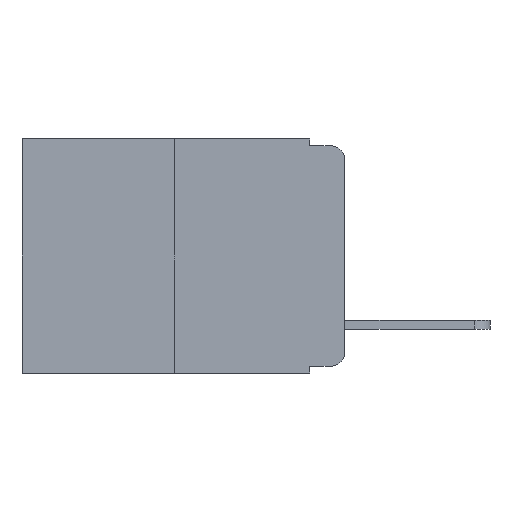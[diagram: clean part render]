
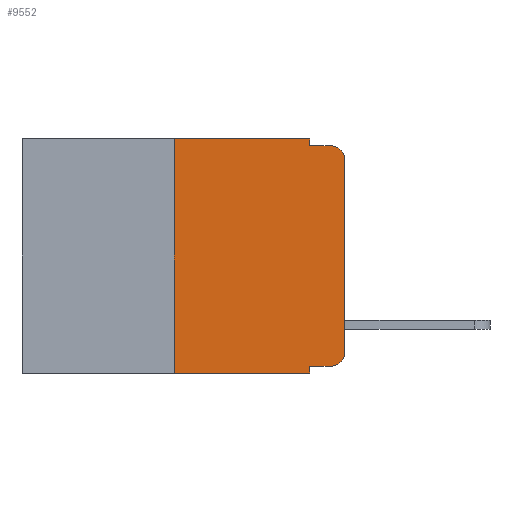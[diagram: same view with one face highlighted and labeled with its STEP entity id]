
A CAD part, left-side view. The second image highlights one B-rep face of the part: STEP entity #9552.
In plain terms, the highlighted planar face has unit normal (-1, 0, 0).
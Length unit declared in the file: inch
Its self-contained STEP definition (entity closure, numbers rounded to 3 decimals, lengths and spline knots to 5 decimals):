
#136 = LINE ( 'NONE', #9930, #23091 ) ;
#436 = CARTESIAN_POINT ( 'NONE',  ( 0., 0.02, -0.333 ) ) ;
#483 = CIRCLE ( 'NONE', #1491, 0.02 ) ;
#1447 = CARTESIAN_POINT ( 'NONE',  ( 0., 0.051, 0. ) ) ;
#1491 = AXIS2_PLACEMENT_3D ( 'NONE', #12486, #14298, #22160 ) ;
#2472 = DIRECTION ( 'NONE',  ( 0., 0., -1. ) ) ;
#2487 = LINE ( 'NONE', #19774, #5887 ) ;
#2876 = VERTEX_POINT ( 'NONE', #5480 ) ;
#3616 = FACE_OUTER_BOUND ( 'NONE', #20516, .T. ) ;
#3927 = VECTOR ( 'NONE', #20649, 39.37008 ) ;
#4208 = VECTOR ( 'NONE', #23397, 39.37008 ) ;
#4296 = EDGE_CURVE ( 'NONE', #2876, #12382, #16126, .T. ) ;
#4303 = DIRECTION ( 'NONE',  ( 0., -1., 0. ) ) ;
#4790 = ORIENTED_EDGE ( 'NONE', *, *, #22300, .F. ) ;
#5338 = CARTESIAN_POINT ( 'NONE',  ( 0., 0.051, -0.01 ) ) ;
#5480 = CARTESIAN_POINT ( 'NONE',  ( 0., 0.051, -0.333 ) ) ;
#5854 = ORIENTED_EDGE ( 'NONE', *, *, #10366, .T. ) ;
#5887 = VECTOR ( 'NONE', #6390, 39.37008 ) ;
#6390 = DIRECTION ( 'NONE',  ( 0., 0., 1. ) ) ;
#6560 = VERTEX_POINT ( 'NONE', #24103 ) ;
#7175 = EDGE_CURVE ( 'NONE', #20776, #17147, #11978, .T. ) ;
#7415 = LINE ( 'NONE', #9196, #9282 ) ;
#7894 = ORIENTED_EDGE ( 'NONE', *, *, #12988, .F. ) ;
#8194 = DIRECTION ( 'NONE',  ( 0., 0., -1. ) ) ;
#8550 = ORIENTED_EDGE ( 'NONE', *, *, #25464, .T. ) ;
#9196 = CARTESIAN_POINT ( 'NONE',  ( 0., 0., 0. ) ) ;
#9223 = CIRCLE ( 'NONE', #21379, 0.02 ) ;
#9281 = CARTESIAN_POINT ( 'NONE',  ( 0., 0.25, 0. ) ) ;
#9282 = VECTOR ( 'NONE', #9374, 39.37008 ) ;
#9374 = DIRECTION ( 'NONE',  ( 0., 0., 1. ) ) ;
#9552 = ADVANCED_FACE ( 'NONE', ( #3616 ), #20704, .F. ) ;
#9930 = CARTESIAN_POINT ( 'NONE',  ( 0., 0.473, -0.343 ) ) ;
#10149 = ORIENTED_EDGE ( 'NONE', *, *, #22702, .T. ) ;
#10366 = EDGE_CURVE ( 'NONE', #14837, #18911, #483, .T. ) ;
#10436 = ORIENTED_EDGE ( 'NONE', *, *, #13458, .T. ) ;
#10779 = CARTESIAN_POINT ( 'NONE',  ( 0., 0.473, 0. ) ) ;
#11978 = LINE ( 'NONE', #23557, #4208 ) ;
#12382 = VERTEX_POINT ( 'NONE', #436 ) ;
#12486 = CARTESIAN_POINT ( 'NONE',  ( 0., 0.02, -0.03 ) ) ;
#12988 = EDGE_CURVE ( 'NONE', #25314, #23221, #2487, .T. ) ;
#13236 = CARTESIAN_POINT ( 'NONE',  ( 0., 0.02, -0.01 ) ) ;
#13458 = EDGE_CURVE ( 'NONE', #6560, #14837, #7415, .T. ) ;
#14298 = DIRECTION ( 'NONE',  ( -1., 0., 0. ) ) ;
#14602 = EDGE_CURVE ( 'NONE', #17147, #18911, #16035, .T. ) ;
#14837 = VERTEX_POINT ( 'NONE', #23226 ) ;
#15304 = ORIENTED_EDGE ( 'NONE', *, *, #7175, .F. ) ;
#15762 = LINE ( 'NONE', #24044, #21383 ) ;
#15894 = CARTESIAN_POINT ( 'NONE',  ( 0., 0.051, -0.343 ) ) ;
#15936 = ORIENTED_EDGE ( 'NONE', *, *, #4296, .T. ) ;
#16035 = LINE ( 'NONE', #16439, #3927 ) ;
#16126 = LINE ( 'NONE', #24629, #20848 ) ;
#16286 = VERTEX_POINT ( 'NONE', #15894 ) ;
#16367 = ORIENTED_EDGE ( 'NONE', *, *, #21676, .F. ) ;
#16439 = CARTESIAN_POINT ( 'NONE',  ( 0., 0.051, -0.01 ) ) ;
#17147 = VERTEX_POINT ( 'NONE', #5338 ) ;
#18271 = VECTOR ( 'NONE', #4303, 39.37008 ) ;
#18911 = VERTEX_POINT ( 'NONE', #13236 ) ;
#19643 = CARTESIAN_POINT ( 'NONE',  ( 0., 0.02, -0.313 ) ) ;
#19774 = CARTESIAN_POINT ( 'NONE',  ( 0., 0.25, 0. ) ) ;
#20014 = DIRECTION ( 'NONE',  ( 0., -1., 0. ) ) ;
#20356 = DIRECTION ( 'NONE',  ( 1., 0., 0. ) ) ;
#20516 = EDGE_LOOP ( 'NONE', ( #10436, #5854, #22734, #15304, #16367, #7894, #8550, #4790, #15936, #10149 ) ) ;
#20649 = DIRECTION ( 'NONE',  ( 0., -1., 0. ) ) ;
#20704 = PLANE ( 'NONE',  #23380 ) ;
#20776 = VERTEX_POINT ( 'NONE', #1447 ) ;
#20848 = VECTOR ( 'NONE', #24373, 39.37008 ) ;
#21379 = AXIS2_PLACEMENT_3D ( 'NONE', #19643, #21577, #21404 ) ;
#21383 = VECTOR ( 'NONE', #8194, 39.37008 ) ;
#21404 = DIRECTION ( 'NONE',  ( 0., 0., -1. ) ) ;
#21577 = DIRECTION ( 'NONE',  ( -1., 0., 0. ) ) ;
#21676 = EDGE_CURVE ( 'NONE', #23221, #20776, #24776, .T. ) ;
#21682 = CARTESIAN_POINT ( 'NONE',  ( 0., 0.25, -0.343 ) ) ;
#21886 = CARTESIAN_POINT ( 'NONE',  ( 0., 0.473, 0. ) ) ;
#22160 = DIRECTION ( 'NONE',  ( 0., 0., -1. ) ) ;
#22300 = EDGE_CURVE ( 'NONE', #2876, #16286, #15762, .T. ) ;
#22702 = EDGE_CURVE ( 'NONE', #12382, #6560, #9223, .T. ) ;
#22734 = ORIENTED_EDGE ( 'NONE', *, *, #14602, .F. ) ;
#23091 = VECTOR ( 'NONE', #20014, 39.37008 ) ;
#23221 = VERTEX_POINT ( 'NONE', #9281 ) ;
#23226 = CARTESIAN_POINT ( 'NONE',  ( 0., 0., -0.03 ) ) ;
#23380 = AXIS2_PLACEMENT_3D ( 'NONE', #10779, #20356, #2472 ) ;
#23397 = DIRECTION ( 'NONE',  ( 0., 0., -1. ) ) ;
#23557 = CARTESIAN_POINT ( 'NONE',  ( 0., 0.051, 0. ) ) ;
#24044 = CARTESIAN_POINT ( 'NONE',  ( 0., 0.051, 0. ) ) ;
#24103 = CARTESIAN_POINT ( 'NONE',  ( 0., 0., -0.313 ) ) ;
#24373 = DIRECTION ( 'NONE',  ( 0., -1., 0. ) ) ;
#24629 = CARTESIAN_POINT ( 'NONE',  ( 0., 0.051, -0.333 ) ) ;
#24776 = LINE ( 'NONE', #21886, #18271 ) ;
#25314 = VERTEX_POINT ( 'NONE', #21682 ) ;
#25464 = EDGE_CURVE ( 'NONE', #25314, #16286, #136, .T. ) ;
